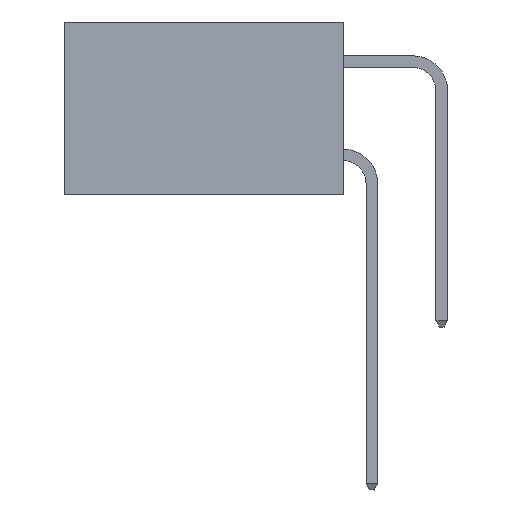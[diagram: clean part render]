
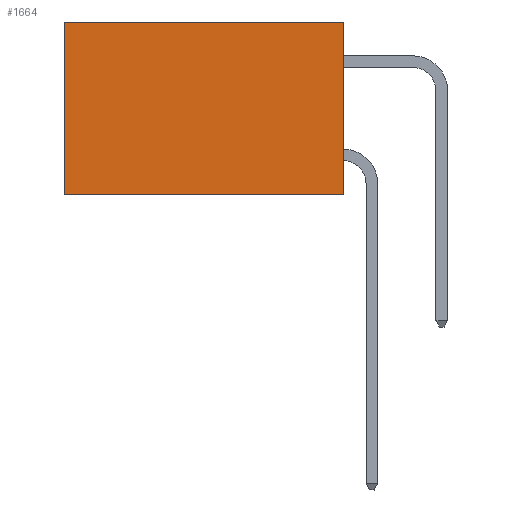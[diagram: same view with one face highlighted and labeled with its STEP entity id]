
A CAD part, left-side view. The second image highlights one B-rep face of the part: STEP entity #1664.
In plain terms, the highlighted planar face has unit normal (-1, 0, 0).
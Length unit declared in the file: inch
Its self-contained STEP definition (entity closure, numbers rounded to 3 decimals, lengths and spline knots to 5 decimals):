
#202 = VERTEX_POINT ( 'NONE', #12338 ) ;
#292 = AXIS2_PLACEMENT_3D ( 'NONE', #22669, #6770, #19941 ) ;
#317 = EDGE_CURVE ( 'NONE', #6835, #202, #13776, .T. ) ;
#618 = EDGE_CURVE ( 'NONE', #20367, #17756, #23008, .T. ) ;
#1622 = LINE ( 'NONE', #5254, #20330 ) ;
#1664 = ADVANCED_FACE ( 'NONE', ( #23224 ), #13873, .F. ) ;
#2592 = ORIENTED_EDGE ( 'NONE', *, *, #317, .F. ) ;
#3191 = CARTESIAN_POINT ( 'NONE',  ( 0.2615, 0., -0.37 ) ) ;
#4920 = EDGE_CURVE ( 'NONE', #20367, #6835, #8069, .T. ) ;
#5254 = CARTESIAN_POINT ( 'NONE',  ( 0.2615, 0.6, -0.37 ) ) ;
#6060 = ORIENTED_EDGE ( 'NONE', *, *, #15566, .T. ) ;
#6770 = DIRECTION ( 'NONE',  ( 1., 0., 0. ) ) ;
#6835 = VERTEX_POINT ( 'NONE', #3191 ) ;
#6930 = VECTOR ( 'NONE', #8034, 39.37008 ) ;
#7244 = DIRECTION ( 'NONE',  ( 0., 0., -1. ) ) ;
#8034 = DIRECTION ( 'NONE',  ( 0., 1., 0. ) ) ;
#8069 = LINE ( 'NONE', #9503, #17152 ) ;
#9503 = CARTESIAN_POINT ( 'NONE',  ( 0.2615, 0., -0.37 ) ) ;
#11036 = DIRECTION ( 'NONE',  ( 0., 0., -1. ) ) ;
#11486 = EDGE_LOOP ( 'NONE', ( #6060, #2592, #20080, #19768 ) ) ;
#12338 = CARTESIAN_POINT ( 'NONE',  ( 0.2615, 0.6, -0.37 ) ) ;
#12561 = CARTESIAN_POINT ( 'NONE',  ( 0.2615, 0., -0.37 ) ) ;
#13193 = VECTOR ( 'NONE', #13225, 39.37008 ) ;
#13225 = DIRECTION ( 'NONE',  ( 0., 1., 0. ) ) ;
#13776 = LINE ( 'NONE', #12561, #13193 ) ;
#13873 = PLANE ( 'NONE',  #292 ) ;
#15566 = EDGE_CURVE ( 'NONE', #17756, #202, #1622, .T. ) ;
#17152 = VECTOR ( 'NONE', #7244, 39.37008 ) ;
#17756 = VERTEX_POINT ( 'NONE', #21285 ) ;
#19010 = CARTESIAN_POINT ( 'NONE',  ( 0.2615, 0., 0. ) ) ;
#19768 = ORIENTED_EDGE ( 'NONE', *, *, #618, .T. ) ;
#19941 = DIRECTION ( 'NONE',  ( 0., 0., -1. ) ) ;
#20080 = ORIENTED_EDGE ( 'NONE', *, *, #4920, .F. ) ;
#20330 = VECTOR ( 'NONE', #11036, 39.37008 ) ;
#20367 = VERTEX_POINT ( 'NONE', #19010 ) ;
#20835 = CARTESIAN_POINT ( 'NONE',  ( 0.2615, 0., 0. ) ) ;
#21285 = CARTESIAN_POINT ( 'NONE',  ( 0.2615, 0.6, 0. ) ) ;
#22669 = CARTESIAN_POINT ( 'NONE',  ( 0.2615, 0., -0.37 ) ) ;
#23008 = LINE ( 'NONE', #20835, #6930 ) ;
#23224 = FACE_OUTER_BOUND ( 'NONE', #11486, .T. ) ;
